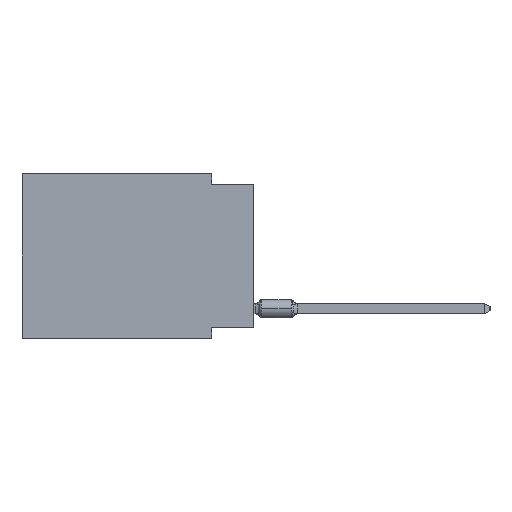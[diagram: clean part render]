
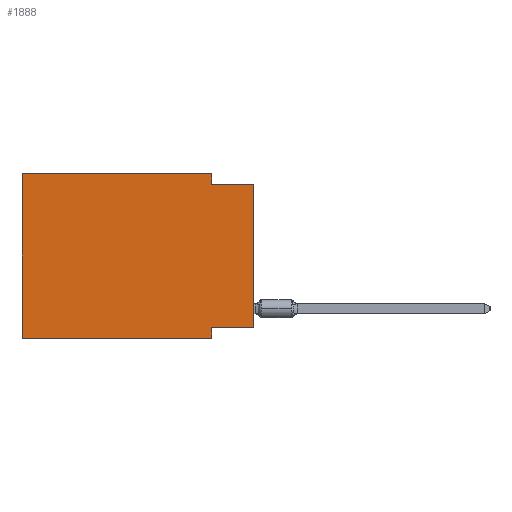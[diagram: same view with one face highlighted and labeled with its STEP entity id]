
A CAD part, left-side view. The second image highlights one B-rep face of the part: STEP entity #1888.
In plain terms, the highlighted planar face has unit normal (-1, 0, 0).
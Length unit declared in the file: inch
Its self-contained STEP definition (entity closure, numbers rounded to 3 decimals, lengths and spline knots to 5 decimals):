
#601 = VERTEX_POINT ( 'NONE', #13668 ) ;
#754 = ORIENTED_EDGE ( 'NONE', *, *, #24062, .F. ) ;
#1673 = FACE_OUTER_BOUND ( 'NONE', #44051, .T. ) ;
#1888 = ADVANCED_FACE ( 'NONE', ( #1673 ), #25277, .F. ) ;
#2279 = DIRECTION ( 'NONE',  ( 1., 0., 0. ) ) ;
#4247 = DIRECTION ( 'NONE',  ( 0., -1., 0. ) ) ;
#4550 = LINE ( 'NONE', #18651, #55588 ) ;
#5834 = VERTEX_POINT ( 'NONE', #22613 ) ;
#6235 = LINE ( 'NONE', #43718, #46338 ) ;
#6417 = VERTEX_POINT ( 'NONE', #10882 ) ;
#7126 = CARTESIAN_POINT ( 'NONE',  ( 0., 0., 0. ) ) ;
#8237 = CARTESIAN_POINT ( 'NONE',  ( 0., 0.55, 0. ) ) ;
#8256 = ORIENTED_EDGE ( 'NONE', *, *, #24722, .F. ) ;
#9861 = CARTESIAN_POINT ( 'NONE',  ( 0., 0., -0.365 ) ) ;
#10882 = CARTESIAN_POINT ( 'NONE',  ( 0., 0.1, -0.365 ) ) ;
#12680 = ORIENTED_EDGE ( 'NONE', *, *, #60525, .F. ) ;
#13668 = CARTESIAN_POINT ( 'NONE',  ( 0., 0.1, -0.025 ) ) ;
#14553 = ORIENTED_EDGE ( 'NONE', *, *, #39358, .F. ) ;
#14583 = LINE ( 'NONE', #8237, #23422 ) ;
#15901 = CARTESIAN_POINT ( 'NONE',  ( 0., 0.55, -0.39 ) ) ;
#16008 = EDGE_CURVE ( 'NONE', #26659, #5834, #38480, .T. ) ;
#16084 = CARTESIAN_POINT ( 'NONE',  ( 0., 0.55, 0. ) ) ;
#16132 = ORIENTED_EDGE ( 'NONE', *, *, #47151, .F. ) ;
#18651 = CARTESIAN_POINT ( 'NONE',  ( 0., 0.1, 0. ) ) ;
#18669 = VECTOR ( 'NONE', #52784, 39.37008 ) ;
#18751 = ORIENTED_EDGE ( 'NONE', *, *, #27997, .F. ) ;
#18884 = CARTESIAN_POINT ( 'NONE',  ( 0., 0.55, -0.39 ) ) ;
#20076 = CARTESIAN_POINT ( 'NONE',  ( 0., 0., -0.365 ) ) ;
#20587 = LINE ( 'NONE', #34127, #36451 ) ;
#22613 = CARTESIAN_POINT ( 'NONE',  ( 0., 0., -0.025 ) ) ;
#23422 = VECTOR ( 'NONE', #4247, 39.37008 ) ;
#24062 = EDGE_CURVE ( 'NONE', #60009, #601, #4550, .T. ) ;
#24575 = CARTESIAN_POINT ( 'NONE',  ( 0., 0.55, 0. ) ) ;
#24722 = EDGE_CURVE ( 'NONE', #601, #5834, #45288, .T. ) ;
#24892 = DIRECTION ( 'NONE',  ( 0., 0., 1. ) ) ;
#25277 = PLANE ( 'NONE',  #46164 ) ;
#26659 = VERTEX_POINT ( 'NONE', #9861 ) ;
#27997 = EDGE_CURVE ( 'NONE', #26659, #6417, #52073, .T. ) ;
#28733 = CARTESIAN_POINT ( 'NONE',  ( 0., 0.1, 0. ) ) ;
#30253 = VECTOR ( 'NONE', #56990, 39.37008 ) ;
#30557 = EDGE_CURVE ( 'NONE', #40906, #37855, #57389, .T. ) ;
#32487 = DIRECTION ( 'NONE',  ( 0., 0., -1. ) ) ;
#33841 = DIRECTION ( 'NONE',  ( 0., 0., 1. ) ) ;
#34127 = CARTESIAN_POINT ( 'NONE',  ( 0., 0.55, 0. ) ) ;
#36451 = VECTOR ( 'NONE', #24892, 39.37008 ) ;
#37855 = VERTEX_POINT ( 'NONE', #52774 ) ;
#38480 = LINE ( 'NONE', #7126, #41156 ) ;
#38499 = DIRECTION ( 'NONE',  ( 0., 0., -1. ) ) ;
#39358 = EDGE_CURVE ( 'NONE', #57325, #60009, #14583, .T. ) ;
#40906 = VERTEX_POINT ( 'NONE', #18884 ) ;
#41156 = VECTOR ( 'NONE', #33841, 39.37008 ) ;
#43718 = CARTESIAN_POINT ( 'NONE',  ( 0., 0.1, -0.39 ) ) ;
#43739 = ORIENTED_EDGE ( 'NONE', *, *, #16008, .T. ) ;
#44051 = EDGE_LOOP ( 'NONE', ( #43739, #8256, #754, #14553, #12680, #60356, #16132, #18751 ) ) ;
#45288 = LINE ( 'NONE', #49292, #58424 ) ;
#46164 = AXIS2_PLACEMENT_3D ( 'NONE', #16084, #2279, #52668 ) ;
#46338 = VECTOR ( 'NONE', #38499, 39.37008 ) ;
#47151 = EDGE_CURVE ( 'NONE', #6417, #37855, #6235, .T. ) ;
#49292 = CARTESIAN_POINT ( 'NONE',  ( 0., 0., -0.025 ) ) ;
#49882 = DIRECTION ( 'NONE',  ( 0., -1., 0. ) ) ;
#52073 = LINE ( 'NONE', #20076, #30253 ) ;
#52668 = DIRECTION ( 'NONE',  ( 0., 0., -1. ) ) ;
#52774 = CARTESIAN_POINT ( 'NONE',  ( 0., 0.1, -0.39 ) ) ;
#52784 = DIRECTION ( 'NONE',  ( 0., -1., 0. ) ) ;
#55588 = VECTOR ( 'NONE', #32487, 39.37008 ) ;
#56990 = DIRECTION ( 'NONE',  ( 0., 1., 0. ) ) ;
#57325 = VERTEX_POINT ( 'NONE', #24575 ) ;
#57389 = LINE ( 'NONE', #15901, #18669 ) ;
#58424 = VECTOR ( 'NONE', #49882, 39.37008 ) ;
#60009 = VERTEX_POINT ( 'NONE', #28733 ) ;
#60356 = ORIENTED_EDGE ( 'NONE', *, *, #30557, .T. ) ;
#60525 = EDGE_CURVE ( 'NONE', #40906, #57325, #20587, .T. ) ;
